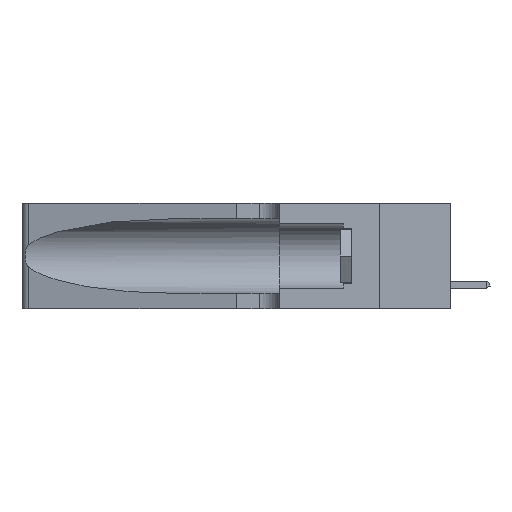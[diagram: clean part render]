
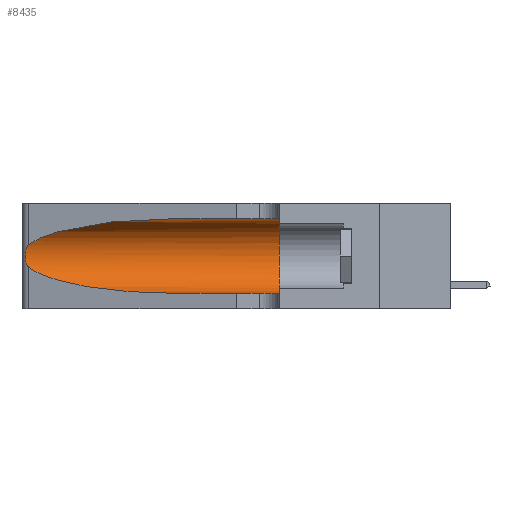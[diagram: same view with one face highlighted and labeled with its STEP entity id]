
A CAD part, left-side view. The second image highlights one B-rep face of the part: STEP entity #8435.
In plain terms, the highlighted cylindrical face has radius 3.308 mm (diameter 6.617 mm), a partial arc.
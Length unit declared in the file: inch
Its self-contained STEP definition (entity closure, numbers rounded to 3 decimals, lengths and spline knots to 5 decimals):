
#398 = CARTESIAN_POINT ( 'NONE',  ( 0.25787, 1.23484, 0.2124 ) ) ;
#588 = CARTESIAN_POINT ( 'NONE',  ( 0.25555, 1.22994, 0.2215 ) ) ;
#1489 = ORIENTED_EDGE ( 'NONE', *, *, #18587, .T. ) ;
#2199 = VERTEX_POINT ( 'NONE', #5691 ) ;
#2507 = CARTESIAN_POINT ( 'NONE',  ( 0.26075, 1.23896, 0.19203 ) ) ;
#2510 = CARTESIAN_POINT ( 'NONE',  ( 0.2373, 1.15595, 0.08982 ) ) ;
#2932 = CARTESIAN_POINT ( 'NONE',  ( 0.18966, 0.96281, 0.31525 ) ) ;
#2958 = VECTOR ( 'NONE', #10547, 39.37008 ) ;
#3543 = DIRECTION ( 'NONE',  ( 0., 0., -1. ) ) ;
#3858 = CARTESIAN_POINT ( 'NONE',  ( 0.1305, 0.72297, 0.31525 ) ) ;
#4342 = AXIS2_PLACEMENT_3D ( 'NONE', #22177, #24468, #26631 ) ;
#5103 = VERTEX_POINT ( 'NONE', #19636 ) ;
#5691 = CARTESIAN_POINT ( 'NONE',  ( 0.1305, 0.35, 0.31525 ) ) ;
#6646 = CARTESIAN_POINT ( 'NONE',  ( 0.25487, 1.22718, 0.22369 ) ) ;
#7038 = ORIENTED_EDGE ( 'NONE', *, *, #22788, .T. ) ;
#7041 = EDGE_LOOP ( 'NONE', ( #10734, #24293, #7038, #1489, #20315, #13514 ) ) ;
#7244 = AXIS2_PLACEMENT_3D ( 'NONE', #12243, #14309, #3543 ) ;
#8171 = DIRECTION ( 'NONE',  ( 0., -1., 0. ) ) ;
#8435 = ADVANCED_FACE ( 'NONE', ( #13188 ), #11892, .F. ) ;
#8643 = CARTESIAN_POINT ( 'NONE',  ( 0.26017, 1.23833, 0.17102 ) ) ;
#8647 = CARTESIAN_POINT ( 'NONE',  ( 0.25487, 1.22718, 0.14631 ) ) ;
#8892 = CARTESIAN_POINT ( 'NONE',  ( 0.2373, 1.15595, 0.28018 ) ) ;
#9006 = CARTESIAN_POINT ( 'NONE',  ( 0.25856, 1.23593, 0.16098 ) ) ;
#10547 = DIRECTION ( 'NONE',  ( 0., -1., 0. ) ) ;
#10734 = ORIENTED_EDGE ( 'NONE', *, *, #26358, .T. ) ;
#11049 =( BOUNDED_CURVE ( )  B_SPLINE_CURVE ( 3, ( #8647, #2510, #14717, #21053 ),
 .UNSPECIFIED., .F., .F. ) 
 B_SPLINE_CURVE_WITH_KNOTS ( ( 4, 4 ),
 ( 3.44316, 4.71239 ),
 .UNSPECIFIED. ) 
 CURVE ( )  GEOMETRIC_REPRESENTATION_ITEM ( )  RATIONAL_B_SPLINE_CURVE ( ( 1., 0.87, 0.87, 1. ) ) 
 REPRESENTATION_ITEM ( '' )  );
#11892 = CYLINDRICAL_SURFACE ( 'NONE', #7244, 0.13025 ) ;
#12243 = CARTESIAN_POINT ( 'NONE',  ( 0.1305, 1.61858, 0.185 ) ) ;
#12506 = VERTEX_POINT ( 'NONE', #26012 ) ;
#12919 = CARTESIAN_POINT ( 'NONE',  ( 0.26018, 1.23835, 0.19895 ) ) ;
#13188 = FACE_OUTER_BOUND ( 'NONE', #7041, .T. ) ;
#13514 = ORIENTED_EDGE ( 'NONE', *, *, #18994, .F. ) ;
#13894 = VERTEX_POINT ( 'NONE', #26033 ) ;
#14309 = DIRECTION ( 'NONE',  ( 0., -1., 0. ) ) ;
#14717 = CARTESIAN_POINT ( 'NONE',  ( 0.18966, 0.96281, 0.05475 ) ) ;
#15088 = CARTESIAN_POINT ( 'NONE',  ( 0.25854, 1.2359, 0.20912 ) ) ;
#15182 = CARTESIAN_POINT ( 'NONE',  ( 0.25789, 1.23486, 0.15765 ) ) ;
#15969 = VECTOR ( 'NONE', #8171, 39.37008 ) ;
#16273 = LINE ( 'NONE', #25813, #15969 ) ;
#16988 = CARTESIAN_POINT ( 'NONE',  ( 0.25555, 1.22993, 0.14849 ) ) ;
#17233 = LINE ( 'NONE', #23074, #2958 ) ;
#17270 = CARTESIAN_POINT ( 'NONE',  ( 0.25487, 1.22718, 0.14631 ) ) ;
#17442 = CARTESIAN_POINT ( 'NONE',  ( 0.25487, 1.22718, 0.22369 ) ) ;
#17594 = CIRCLE ( 'NONE', #4342, 0.13025 ) ;
#17909 = B_SPLINE_CURVE_WITH_KNOTS ( 'NONE', 3,
 ( #6646, #588, #23546, #398, #15088, #12919, #2507, #21517, #8643, #9006, #15182, #21231, #16988, #17270 ),
 .UNSPECIFIED., .F., .F.,
 ( 4, 2, 2, 2, 2, 2, 4 ),
 ( 0., 0.00027, 0.00053, 0.00107, 0.0016, 0.00187, 0.00214 ),
 .UNSPECIFIED. ) ;
#18587 = EDGE_CURVE ( 'NONE', #12506, #13894, #16273, .T. ) ;
#18994 = EDGE_CURVE ( 'NONE', #24189, #2199, #17233, .T. ) ;
#19038 = EDGE_CURVE ( 'NONE', #21715, #5103, #17909, .T. ) ;
#19297 = CARTESIAN_POINT ( 'NONE',  ( 0.1305, 0.72297, 0.31525 ) ) ;
#19636 = CARTESIAN_POINT ( 'NONE',  ( 0.25487, 1.22718, 0.14631 ) ) ;
#20315 = ORIENTED_EDGE ( 'NONE', *, *, #23999, .F. ) ;
#21053 = CARTESIAN_POINT ( 'NONE',  ( 0.1305, 0.72297, 0.05475 ) ) ;
#21231 = CARTESIAN_POINT ( 'NONE',  ( 0.25639, 1.23186, 0.15144 ) ) ;
#21517 = CARTESIAN_POINT ( 'NONE',  ( 0.26075, 1.23896, 0.178 ) ) ;
#21715 = VERTEX_POINT ( 'NONE', #23976 ) ;
#22177 = CARTESIAN_POINT ( 'NONE',  ( 0.1305, 0.35, 0.185 ) ) ;
#22788 = EDGE_CURVE ( 'NONE', #5103, #12506, #11049, .T. ) ;
#23074 = CARTESIAN_POINT ( 'NONE',  ( 0.1305, 1.61858, 0.31525 ) ) ;
#23546 = CARTESIAN_POINT ( 'NONE',  ( 0.25639, 1.23184, 0.21858 ) ) ;
#23639 =( BOUNDED_CURVE ( )  B_SPLINE_CURVE ( 3, ( #19297, #2932, #8892, #17442 ),
 .UNSPECIFIED., .F., .T. ) 
 B_SPLINE_CURVE_WITH_KNOTS ( ( 4, 4 ),
 ( 1.5708, 2.84003 ),
 .UNSPECIFIED. ) 
 CURVE ( )  GEOMETRIC_REPRESENTATION_ITEM ( )  RATIONAL_B_SPLINE_CURVE ( ( 1., 0.87, 0.87, 1. ) ) 
 REPRESENTATION_ITEM ( '' )  );
#23976 = CARTESIAN_POINT ( 'NONE',  ( 0.25487, 1.22718, 0.22369 ) ) ;
#23999 = EDGE_CURVE ( 'NONE', #2199, #13894, #17594, .T. ) ;
#24189 = VERTEX_POINT ( 'NONE', #3858 ) ;
#24293 = ORIENTED_EDGE ( 'NONE', *, *, #19038, .T. ) ;
#24468 = DIRECTION ( 'NONE',  ( 0., 1., 0. ) ) ;
#25813 = CARTESIAN_POINT ( 'NONE',  ( 0.1305, 1.61858, 0.05475 ) ) ;
#26012 = CARTESIAN_POINT ( 'NONE',  ( 0.1305, 0.72297, 0.05475 ) ) ;
#26033 = CARTESIAN_POINT ( 'NONE',  ( 0.1305, 0.35, 0.05475 ) ) ;
#26358 = EDGE_CURVE ( 'NONE', #24189, #21715, #23639, .T. ) ;
#26631 = DIRECTION ( 'NONE',  ( 0., 0., 1. ) ) ;
